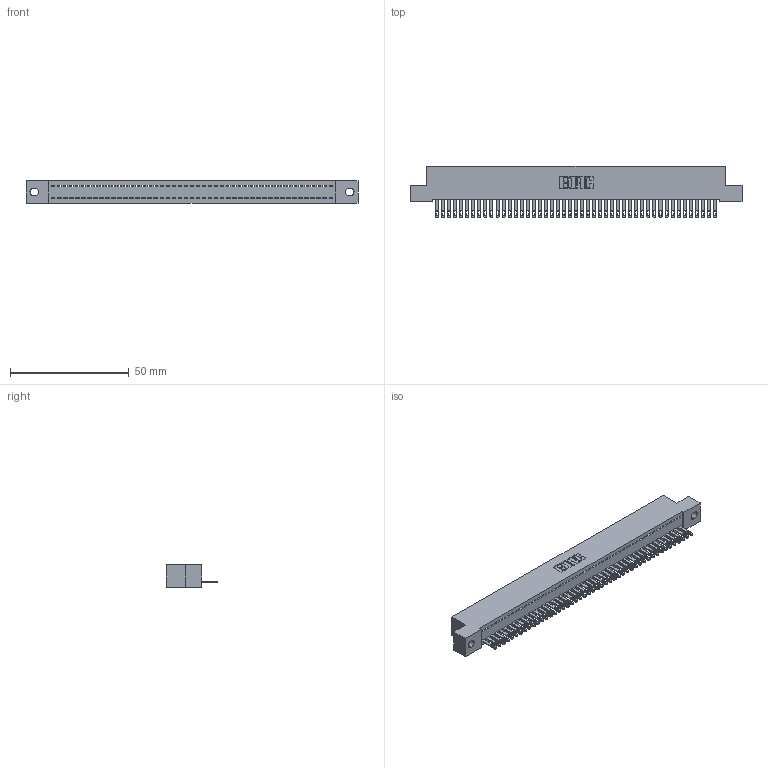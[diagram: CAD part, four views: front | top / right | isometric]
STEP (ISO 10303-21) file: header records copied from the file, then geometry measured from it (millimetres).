
FILE_DESCRIPTION (( 'STEP AP203' ), '1' );
FILE_NAME ('892-047-500-102.STEP', '2020-09-21T17:22:23', ( '' ), ( '' ), 'SwSTEP 2.0', 'SolidWorks 2020', '' );
FILE_SCHEMA (( 'CONFIG_CONTROL_DESIGN' ));
Length unit declared in the file: inch
Products named in the file (3): 892-047-500-102; 842 Part_.128 Slot; 345-292-001_345-293-100
Assembly tree (48 placements, depth 2):
  892-047-500-102
    842 Part_.128 Slot
    345-292-001_345-293-100  x47
Bounding box: 139.7 x 21.85 x 9.4 mm (x, y, z)
Volume: 12244.3 mm3; surface area: 17925.6 mm2
Topology: 48 solids, 48 shells, 2652 faces, 8207 edges, 5470 vertices
Faces by surface type: plane 1762, cylinder 890
Entity records: 28019 total; most frequent: CARTESIAN_POINT 4839, ORIENTED_EDGE 4822, DIRECTION 4073, EDGE_CURVE 2411, VECTOR 2279, LINE 2279, VERTEX_POINT 1606, AXIS2_PLACEMENT_3D 897
